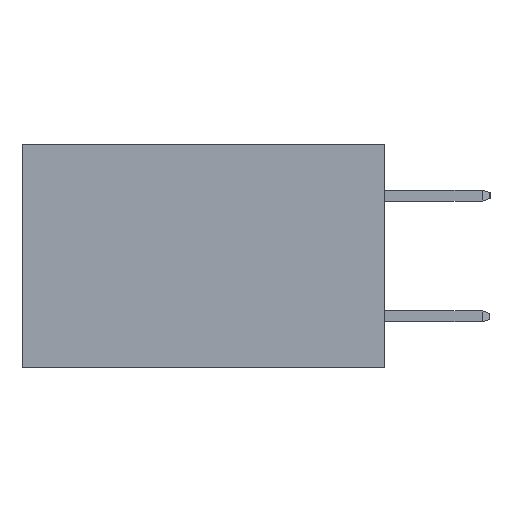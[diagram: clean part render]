
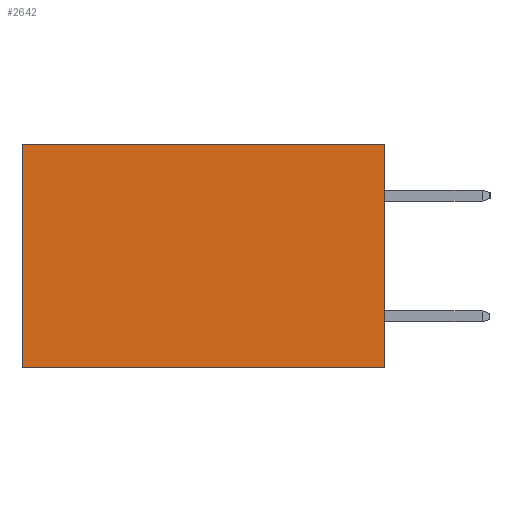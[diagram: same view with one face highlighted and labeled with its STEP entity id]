
A CAD part, left-side view. The second image highlights one B-rep face of the part: STEP entity #2642.
In plain terms, the highlighted planar face has unit normal (-1, 0, 0).
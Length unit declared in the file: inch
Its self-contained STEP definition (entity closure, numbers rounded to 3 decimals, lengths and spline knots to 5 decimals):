
#242 = CARTESIAN_POINT ( 'NONE',  ( 0.298, 0., 0. ) ) ;
#305 = AXIS2_PLACEMENT_3D ( 'NONE', #4252, #5153, #8345 ) ;
#1514 = ORIENTED_EDGE ( 'NONE', *, *, #9126, .T. ) ;
#1531 = LINE ( 'NONE', #5510, #6658 ) ;
#1597 = CARTESIAN_POINT ( 'NONE',  ( 0.298, 0., 0. ) ) ;
#2000 = DIRECTION ( 'NONE',  ( 0., 1., 0. ) ) ;
#2520 = DIRECTION ( 'NONE',  ( 0., 1., 0. ) ) ;
#2642 = ADVANCED_FACE ( 'NONE', ( #9598 ), #4013, .F. ) ;
#2676 = EDGE_CURVE ( 'NONE', #3397, #2920, #1531, .T. ) ;
#2794 = EDGE_CURVE ( 'NONE', #11088, #2920, #7071, .T. ) ;
#2920 = VERTEX_POINT ( 'NONE', #7632 ) ;
#3397 = VERTEX_POINT ( 'NONE', #4968 ) ;
#4013 = PLANE ( 'NONE',  #305 ) ;
#4252 = CARTESIAN_POINT ( 'NONE',  ( 0.298, 0., 0. ) ) ;
#4415 = EDGE_CURVE ( 'NONE', #10668, #3397, #10370, .T. ) ;
#4968 = CARTESIAN_POINT ( 'NONE',  ( 0.298, 0., -0.37 ) ) ;
#5153 = DIRECTION ( 'NONE',  ( 1., 0., 0. ) ) ;
#5510 = CARTESIAN_POINT ( 'NONE',  ( 0.298, 0., -0.37 ) ) ;
#6478 = CARTESIAN_POINT ( 'NONE',  ( 0.298, 0.6, 0. ) ) ;
#6658 = VECTOR ( 'NONE', #2520, 39.37008 ) ;
#7071 = LINE ( 'NONE', #7573, #9465 ) ;
#7143 = EDGE_LOOP ( 'NONE', ( #9410, #10535, #11498, #1514 ) ) ;
#7400 = LINE ( 'NONE', #8331, #9497 ) ;
#7573 = CARTESIAN_POINT ( 'NONE',  ( 0.298, 0.6, 0. ) ) ;
#7632 = CARTESIAN_POINT ( 'NONE',  ( 0.298, 0.6, -0.37 ) ) ;
#8331 = CARTESIAN_POINT ( 'NONE',  ( 0.298, 0., 0. ) ) ;
#8345 = DIRECTION ( 'NONE',  ( 0., 0., -1. ) ) ;
#9126 = EDGE_CURVE ( 'NONE', #10668, #11088, #7400, .T. ) ;
#9410 = ORIENTED_EDGE ( 'NONE', *, *, #2794, .T. ) ;
#9465 = VECTOR ( 'NONE', #10532, 39.37008 ) ;
#9497 = VECTOR ( 'NONE', #2000, 39.37008 ) ;
#9598 = FACE_OUTER_BOUND ( 'NONE', #7143, .T. ) ;
#10370 = LINE ( 'NONE', #242, #10642 ) ;
#10532 = DIRECTION ( 'NONE',  ( 0., 0., -1. ) ) ;
#10535 = ORIENTED_EDGE ( 'NONE', *, *, #2676, .F. ) ;
#10642 = VECTOR ( 'NONE', #10793, 39.37008 ) ;
#10668 = VERTEX_POINT ( 'NONE', #1597 ) ;
#10793 = DIRECTION ( 'NONE',  ( 0., 0., -1. ) ) ;
#11088 = VERTEX_POINT ( 'NONE', #6478 ) ;
#11498 = ORIENTED_EDGE ( 'NONE', *, *, #4415, .F. ) ;
